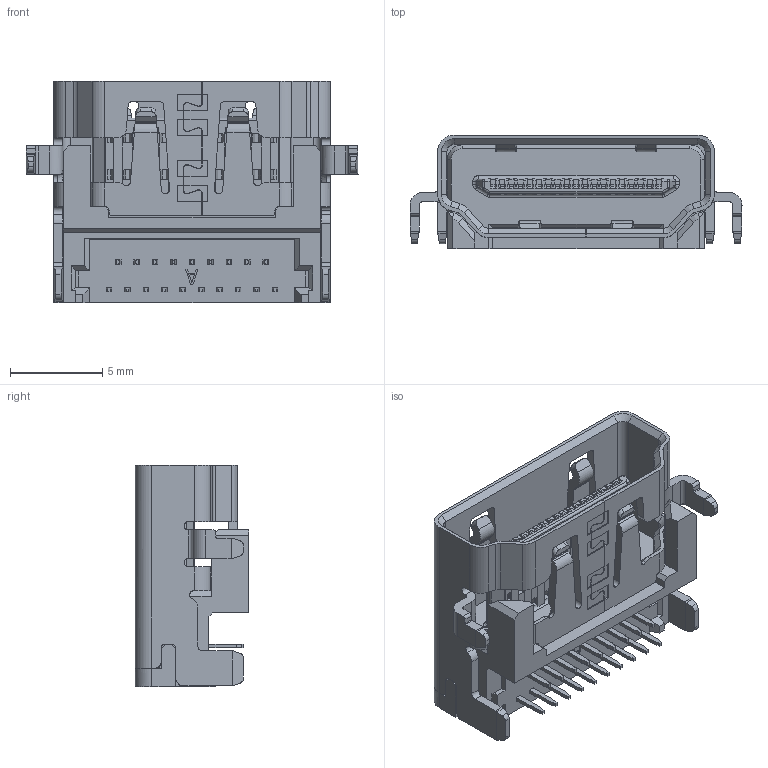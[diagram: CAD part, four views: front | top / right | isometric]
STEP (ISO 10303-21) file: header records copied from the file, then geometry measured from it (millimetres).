
FILE_DESCRIPTION (( 'STEP AP214' ), '1' );
FILE_NAME ('694C119-153-011.STEP', '2021-01-13T14:49:40', ( '' ), ( '' ), 'SwSTEP 2.0', 'SolidWorks 2020', '' );
FILE_SCHEMA (( 'AUTOMOTIVE_DESIGN' ));
Length unit declared in the file: millimetre
Products named in the file (6): 694C119-153-011; Contact Upper 694C119-X53-01X; Contact Lower 694C119-X53-01X; Insulator2 694C119-X53-01X; Insulator1 694C119-X53-01X; Shell 694C119-X53-01X
Assembly tree (22 placements, depth 2):
  694C119-153-011
    Insulator1 694C119-X53-01X
    Contact Upper 694C119-X53-01X  x10
    Contact Lower 694C119-X53-01X  x9
    Insulator2 694C119-X53-01X
    Shell 694C119-X53-01X
Bounding box: 18 x 6.16 x 12 mm (x, y, z)
Volume: 414.8 mm3; surface area: 1720.4 mm2
Topology: 22 solids, 22 shells, 3094 faces, 8892 edges, 5752 vertices
Faces by surface type: plane 2147, cylinder 896, bspline 26, cone 25
Entity records: 78784 total; most frequent: CARTESIAN_POINT 17933, ORIENTED_EDGE 13602, DIRECTION 11371, EDGE_CURVE 6801, VECTOR 4761, LINE 4761, VERTEX_POINT 4358, AXIS2_PLACEMENT_3D 3305
